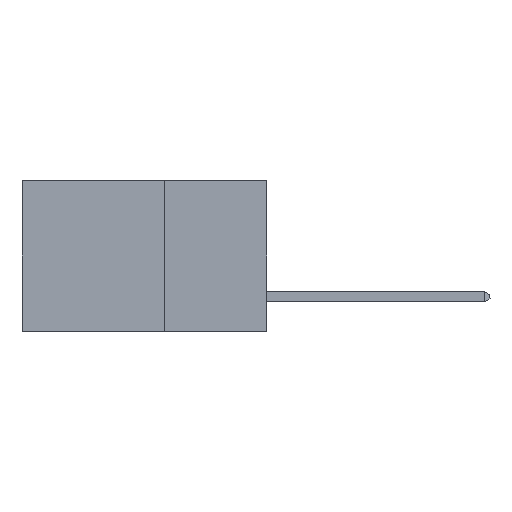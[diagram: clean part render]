
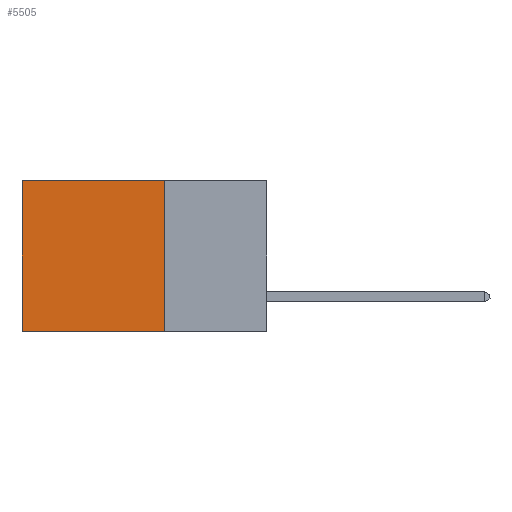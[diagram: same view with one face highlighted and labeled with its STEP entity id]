
A CAD part, left-side view. The second image highlights one B-rep face of the part: STEP entity #5505.
In plain terms, the highlighted planar face has unit normal (-1, 0, 0).
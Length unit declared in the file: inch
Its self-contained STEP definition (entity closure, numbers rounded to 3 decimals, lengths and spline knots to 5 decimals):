
#64 = EDGE_LOOP ( 'NONE', ( #7988, #581, #8247, #8514 ) ) ;
#575 = VECTOR ( 'NONE', #2108, 39.37008 ) ;
#581 = ORIENTED_EDGE ( 'NONE', *, *, #1014, .F. ) ;
#1014 = EDGE_CURVE ( 'NONE', #2658, #10197, #9172, .T. ) ;
#1207 = CARTESIAN_POINT ( 'NONE',  ( 0.2875, 0.25, 0. ) ) ;
#1247 = DIRECTION ( 'NONE',  ( 0., 0., -1. ) ) ;
#1336 = EDGE_CURVE ( 'NONE', #9236, #2658, #3162, .T. ) ;
#1560 = FACE_OUTER_BOUND ( 'NONE', #64, .T. ) ;
#1949 = CARTESIAN_POINT ( 'NONE',  ( 0.2875, 0.25, 0. ) ) ;
#2108 = DIRECTION ( 'NONE',  ( 0., 0., -1. ) ) ;
#2658 = VERTEX_POINT ( 'NONE', #8209 ) ;
#2735 = CARTESIAN_POINT ( 'NONE',  ( 0.2875, 0.25, 0. ) ) ;
#2779 = CARTESIAN_POINT ( 'NONE',  ( 0.2875, 0.6, 0. ) ) ;
#3081 = CARTESIAN_POINT ( 'NONE',  ( 0.2875, 0.25, -0.37 ) ) ;
#3162 = LINE ( 'NONE', #1949, #575 ) ;
#3265 = VECTOR ( 'NONE', #3722, 39.37008 ) ;
#3376 = DIRECTION ( 'NONE',  ( 0., 1., 0. ) ) ;
#3722 = DIRECTION ( 'NONE',  ( 0., 1., 0. ) ) ;
#3881 = VECTOR ( 'NONE', #1247, 39.37008 ) ;
#4098 = EDGE_CURVE ( 'NONE', #6576, #10197, #11029, .T. ) ;
#4353 = CARTESIAN_POINT ( 'NONE',  ( 0.2875, 0.6, 0. ) ) ;
#5505 = ADVANCED_FACE ( 'NONE', ( #1560 ), #7862, .F. ) ;
#6576 = VERTEX_POINT ( 'NONE', #2779 ) ;
#7681 = DIRECTION ( 'NONE',  ( 0., 0., -1. ) ) ;
#7693 = DIRECTION ( 'NONE',  ( 1., 0., 0. ) ) ;
#7862 = PLANE ( 'NONE',  #9323 ) ;
#7988 = ORIENTED_EDGE ( 'NONE', *, *, #4098, .T. ) ;
#8003 = CARTESIAN_POINT ( 'NONE',  ( 0.2875, 0.25, 0. ) ) ;
#8209 = CARTESIAN_POINT ( 'NONE',  ( 0.2875, 0.25, -0.37 ) ) ;
#8247 = ORIENTED_EDGE ( 'NONE', *, *, #1336, .F. ) ;
#8514 = ORIENTED_EDGE ( 'NONE', *, *, #10130, .T. ) ;
#9172 = LINE ( 'NONE', #3081, #11076 ) ;
#9236 = VERTEX_POINT ( 'NONE', #1207 ) ;
#9323 = AXIS2_PLACEMENT_3D ( 'NONE', #8003, #7693, #7681 ) ;
#10130 = EDGE_CURVE ( 'NONE', #9236, #6576, #10529, .T. ) ;
#10197 = VERTEX_POINT ( 'NONE', #10990 ) ;
#10529 = LINE ( 'NONE', #2735, #3265 ) ;
#10990 = CARTESIAN_POINT ( 'NONE',  ( 0.2875, 0.6, -0.37 ) ) ;
#11029 = LINE ( 'NONE', #4353, #3881 ) ;
#11076 = VECTOR ( 'NONE', #3376, 39.37008 ) ;
